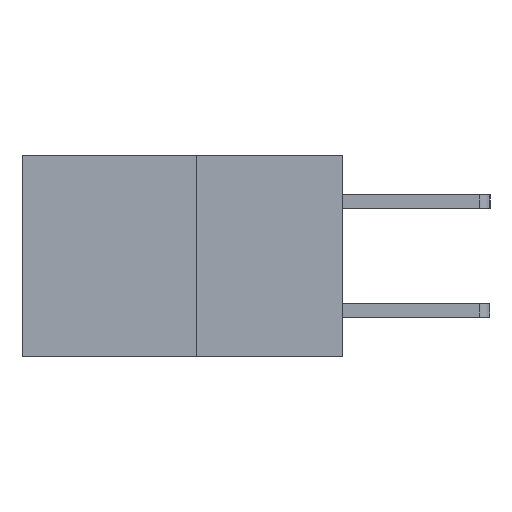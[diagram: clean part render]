
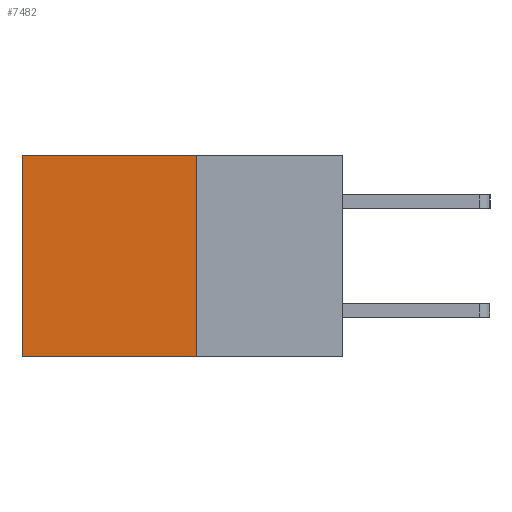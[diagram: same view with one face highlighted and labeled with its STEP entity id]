
A CAD part, left-side view. The second image highlights one B-rep face of the part: STEP entity #7482.
In plain terms, the highlighted planar face has unit normal (-1, 0, 0).
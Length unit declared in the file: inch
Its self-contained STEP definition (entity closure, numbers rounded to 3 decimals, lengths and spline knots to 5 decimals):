
#74 = CARTESIAN_POINT ( 'NONE',  ( 0.277, 0.27, -0.37 ) ) ;
#193 = CARTESIAN_POINT ( 'NONE',  ( 0.277, 0.27, -0.37 ) ) ;
#434 = VERTEX_POINT ( 'NONE', #4321 ) ;
#1667 = CARTESIAN_POINT ( 'NONE',  ( 0.277, 0.59, 0. ) ) ;
#2050 = ORIENTED_EDGE ( 'NONE', *, *, #11247, .T. ) ;
#2431 = EDGE_LOOP ( 'NONE', ( #11473, #5144, #8368, #2050 ) ) ;
#2624 = DIRECTION ( 'NONE',  ( 0., 0., -1. ) ) ;
#2691 = DIRECTION ( 'NONE',  ( 1., 0., 0. ) ) ;
#2779 = DIRECTION ( 'NONE',  ( 0., 0., -1. ) ) ;
#2819 = CARTESIAN_POINT ( 'NONE',  ( 0.277, 0.27, -0.37 ) ) ;
#2884 = PLANE ( 'NONE',  #4472 ) ;
#3300 = EDGE_CURVE ( 'NONE', #434, #9072, #3875, .T. ) ;
#3875 = LINE ( 'NONE', #193, #8363 ) ;
#4210 = LINE ( 'NONE', #6182, #6327 ) ;
#4321 = CARTESIAN_POINT ( 'NONE',  ( 0.277, 0.27, -0.37 ) ) ;
#4472 = AXIS2_PLACEMENT_3D ( 'NONE', #2819, #2691, #2624 ) ;
#4731 = LINE ( 'NONE', #74, #11059 ) ;
#4813 = VERTEX_POINT ( 'NONE', #9549 ) ;
#5144 = ORIENTED_EDGE ( 'NONE', *, *, #3300, .F. ) ;
#5385 = EDGE_CURVE ( 'NONE', #4813, #434, #4731, .T. ) ;
#6182 = CARTESIAN_POINT ( 'NONE',  ( 0.277, 0.27, 0. ) ) ;
#6327 = VECTOR ( 'NONE', #7133, 39.37008 ) ;
#7133 = DIRECTION ( 'NONE',  ( 0., 1., 0. ) ) ;
#7230 = DIRECTION ( 'NONE',  ( 0., 1., 0. ) ) ;
#7482 = ADVANCED_FACE ( 'NONE', ( #10206 ), #2884, .F. ) ;
#7590 = VERTEX_POINT ( 'NONE', #1667 ) ;
#7674 = DIRECTION ( 'NONE',  ( 0., 0., -1. ) ) ;
#8305 = VECTOR ( 'NONE', #2779, 39.37008 ) ;
#8363 = VECTOR ( 'NONE', #7230, 39.37008 ) ;
#8368 = ORIENTED_EDGE ( 'NONE', *, *, #5385, .F. ) ;
#8566 = LINE ( 'NONE', #9844, #8305 ) ;
#9072 = VERTEX_POINT ( 'NONE', #10547 ) ;
#9549 = CARTESIAN_POINT ( 'NONE',  ( 0.277, 0.27, 0. ) ) ;
#9844 = CARTESIAN_POINT ( 'NONE',  ( 0.277, 0.59, -0.37 ) ) ;
#9964 = EDGE_CURVE ( 'NONE', #7590, #9072, #8566, .T. ) ;
#10206 = FACE_OUTER_BOUND ( 'NONE', #2431, .T. ) ;
#10547 = CARTESIAN_POINT ( 'NONE',  ( 0.277, 0.59, -0.37 ) ) ;
#11059 = VECTOR ( 'NONE', #7674, 39.37008 ) ;
#11247 = EDGE_CURVE ( 'NONE', #4813, #7590, #4210, .T. ) ;
#11473 = ORIENTED_EDGE ( 'NONE', *, *, #9964, .T. ) ;
